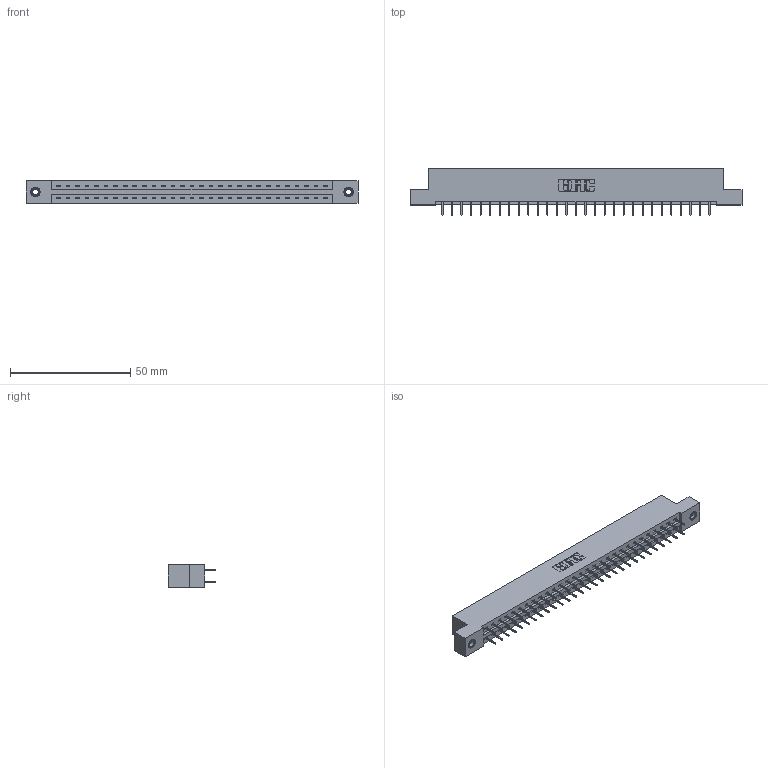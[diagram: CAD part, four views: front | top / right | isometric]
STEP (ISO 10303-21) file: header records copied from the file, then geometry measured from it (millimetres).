
FILE_DESCRIPTION (( 'STEP AP203' ), '1' );
FILE_NAME ('387-058-524-207.STEP', '2018-09-21T01:15:11', ( '' ), ( '' ), 'SwSTEP 2.0', 'SolidWorks 2016', '' );
FILE_SCHEMA (( 'CONFIG_CONTROL_DESIGN' ));
Length unit declared in the file: inch
Products named in the file (4): 337 Part_Flush Mounting Lugs - 0.156 Dia-TI; 345-292-001_345-293-124; 345-250-001_345-250-005-103; 387-058-524-207
Assembly tree (61 placements, depth 2):
  387-058-524-207
    337 Part_Flush Mounting Lugs - 0.156 Dia-TI
    345-292-001_345-293-124  x58
    345-250-001_345-250-005-103  x2
Bounding box: 137.92 x 19.69 x 9.4 mm (x, y, z)
Volume: 14261 mm3; surface area: 15759.9 mm2
Topology: 61 solids, 61 shells, 3538 faces, 10017 edges, 6438 vertices
Faces by surface type: plane 2654, cylinder 868, cone 12, torus 4
Entity records: 25426 total; most frequent: CARTESIAN_POINT 4273, ORIENTED_EDGE 4202, DIRECTION 3691, EDGE_CURVE 2101, LINE 1957, VECTOR 1957, VERTEX_POINT 1392, AXIS2_PLACEMENT_3D 867
